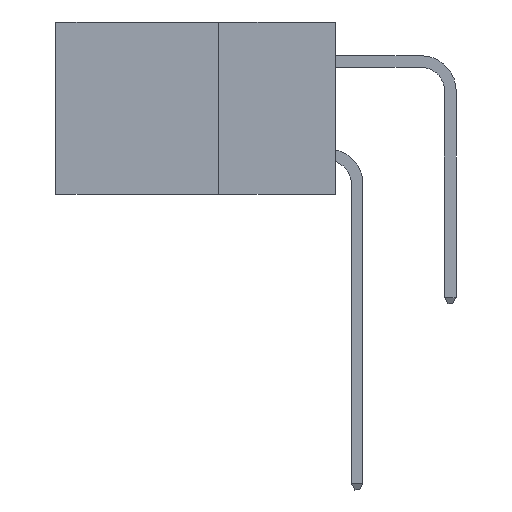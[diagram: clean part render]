
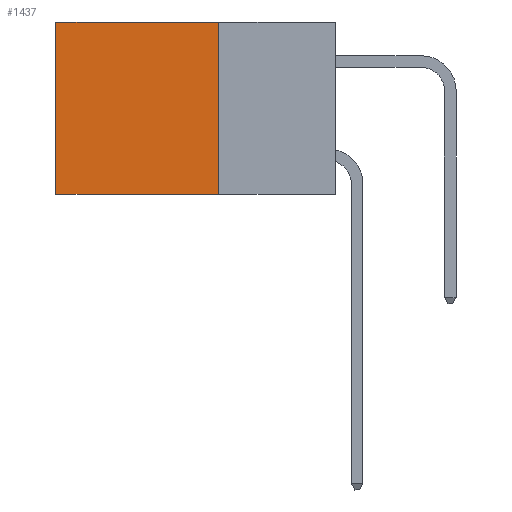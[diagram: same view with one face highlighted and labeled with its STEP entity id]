
A CAD part, left-side view. The second image highlights one B-rep face of the part: STEP entity #1437.
In plain terms, the highlighted planar face has unit normal (-1, 0, 0).
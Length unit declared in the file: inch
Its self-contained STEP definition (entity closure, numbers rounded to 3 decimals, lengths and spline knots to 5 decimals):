
#394 = CARTESIAN_POINT ( 'NONE',  ( 0.2875, 0.25, 0. ) ) ;
#927 = LINE ( 'NONE', #4852, #12915 ) ;
#1246 = VERTEX_POINT ( 'NONE', #3167 ) ;
#1437 = ADVANCED_FACE ( 'NONE', ( #24806 ), #15841, .F. ) ;
#1748 = DIRECTION ( 'NONE',  ( 0., 0., -1. ) ) ;
#2402 = EDGE_CURVE ( 'NONE', #9179, #23386, #19392, .T. ) ;
#3014 = VECTOR ( 'NONE', #25825, 39.37008 ) ;
#3167 = CARTESIAN_POINT ( 'NONE',  ( 0.2875, 0.25, -0.37 ) ) ;
#4657 = DIRECTION ( 'NONE',  ( 0., 1., 0. ) ) ;
#4803 = EDGE_CURVE ( 'NONE', #11418, #1246, #927, .T. ) ;
#4852 = CARTESIAN_POINT ( 'NONE',  ( 0.2875, 0.25, 0. ) ) ;
#5710 = CARTESIAN_POINT ( 'NONE',  ( 0.2875, 0.6, 0. ) ) ;
#7124 = EDGE_LOOP ( 'NONE', ( #9669, #10345, #7462, #23501 ) ) ;
#7462 = ORIENTED_EDGE ( 'NONE', *, *, #4803, .F. ) ;
#7663 = VECTOR ( 'NONE', #1748, 39.37008 ) ;
#9179 = VERTEX_POINT ( 'NONE', #19566 ) ;
#9669 = ORIENTED_EDGE ( 'NONE', *, *, #2402, .T. ) ;
#9816 = DIRECTION ( 'NONE',  ( 0., 0., -1. ) ) ;
#10345 = ORIENTED_EDGE ( 'NONE', *, *, #19077, .F. ) ;
#10510 = EDGE_CURVE ( 'NONE', #11418, #9179, #19636, .T. ) ;
#11418 = VERTEX_POINT ( 'NONE', #25062 ) ;
#12915 = VECTOR ( 'NONE', #14808, 39.37008 ) ;
#14808 = DIRECTION ( 'NONE',  ( 0., 0., -1. ) ) ;
#15841 = PLANE ( 'NONE',  #17935 ) ;
#17935 = AXIS2_PLACEMENT_3D ( 'NONE', #19846, #21937, #9816 ) ;
#18305 = VECTOR ( 'NONE', #4657, 39.37008 ) ;
#19077 = EDGE_CURVE ( 'NONE', #1246, #23386, #23588, .T. ) ;
#19392 = LINE ( 'NONE', #5710, #7663 ) ;
#19566 = CARTESIAN_POINT ( 'NONE',  ( 0.2875, 0.6, 0. ) ) ;
#19636 = LINE ( 'NONE', #394, #18305 ) ;
#19846 = CARTESIAN_POINT ( 'NONE',  ( 0.2875, 0.25, 0. ) ) ;
#20194 = CARTESIAN_POINT ( 'NONE',  ( 0.2875, 0.6, -0.37 ) ) ;
#21937 = DIRECTION ( 'NONE',  ( 1., 0., 0. ) ) ;
#23386 = VERTEX_POINT ( 'NONE', #20194 ) ;
#23501 = ORIENTED_EDGE ( 'NONE', *, *, #10510, .T. ) ;
#23588 = LINE ( 'NONE', #25737, #3014 ) ;
#24806 = FACE_OUTER_BOUND ( 'NONE', #7124, .T. ) ;
#25062 = CARTESIAN_POINT ( 'NONE',  ( 0.2875, 0.25, 0. ) ) ;
#25737 = CARTESIAN_POINT ( 'NONE',  ( 0.2875, 0.25, -0.37 ) ) ;
#25825 = DIRECTION ( 'NONE',  ( 0., 1., 0. ) ) ;
